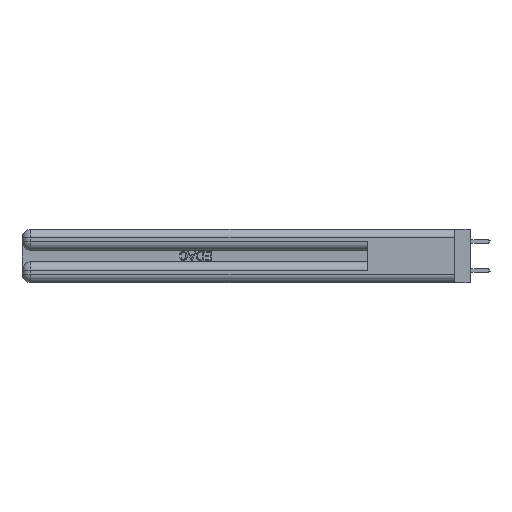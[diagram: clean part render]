
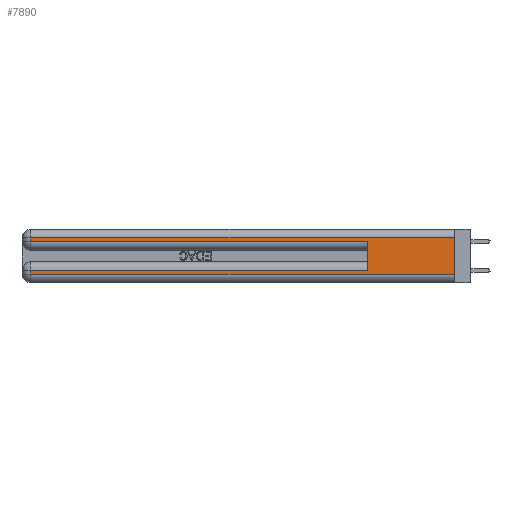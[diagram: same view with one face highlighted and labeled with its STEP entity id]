
A CAD part, left-side view. The second image highlights one B-rep face of the part: STEP entity #7890.
In plain terms, the highlighted planar face has unit normal (-1, 0, 0).
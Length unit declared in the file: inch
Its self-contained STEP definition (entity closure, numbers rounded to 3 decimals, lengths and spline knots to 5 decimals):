
#1104 = VECTOR ( 'NONE', #36062, 39.37008 ) ;
#1747 = LINE ( 'NONE', #12879, #42386 ) ;
#1796 = LINE ( 'NONE', #11357, #41329 ) ;
#2652 = DIRECTION ( 'NONE',  ( 0., 0., -1. ) ) ;
#4220 = DIRECTION ( 'NONE',  ( 0., 0., 1. ) ) ;
#4617 = VECTOR ( 'NONE', #34123, 39.37008 ) ;
#5844 = PLANE ( 'NONE',  #22096 ) ;
#7332 = LINE ( 'NONE', #20601, #35048 ) ;
#7825 = VERTEX_POINT ( 'NONE', #23229 ) ;
#7890 = ADVANCED_FACE ( 'NONE', ( #29315 ), #5844, .F. ) ;
#8463 = LINE ( 'NONE', #35904, #1104 ) ;
#9007 = DIRECTION ( 'NONE',  ( 0., 0., -1. ) ) ;
#10583 = VERTEX_POINT ( 'NONE', #43640 ) ;
#11357 = CARTESIAN_POINT ( 'NONE',  ( 0., 0., 0.085 ) ) ;
#11877 = CARTESIAN_POINT ( 'NONE',  ( 0., 2.94, 0.31 ) ) ;
#12556 = VERTEX_POINT ( 'NONE', #19531 ) ;
#12879 = CARTESIAN_POINT ( 'NONE',  ( 0., 0., 0.06 ) ) ;
#13426 = CARTESIAN_POINT ( 'NONE',  ( 0., 2.94, 0.085 ) ) ;
#14580 = ORIENTED_EDGE ( 'NONE', *, *, #31285, .T. ) ;
#15949 = ORIENTED_EDGE ( 'NONE', *, *, #45299, .F. ) ;
#16547 = LINE ( 'NONE', #38335, #45295 ) ;
#16735 = LINE ( 'NONE', #44305, #24644 ) ;
#17589 = EDGE_LOOP ( 'NONE', ( #15949, #14580, #35739, #26952, #22542, #34376, #24876, #18691 ) ) ;
#18691 = ORIENTED_EDGE ( 'NONE', *, *, #38972, .T. ) ;
#19492 = LINE ( 'NONE', #37578, #43164 ) ;
#19531 = CARTESIAN_POINT ( 'NONE',  ( 0., 0., 0.31 ) ) ;
#20601 = CARTESIAN_POINT ( 'NONE',  ( 0., 2.94, 0.37 ) ) ;
#21417 = VERTEX_POINT ( 'NONE', #11877 ) ;
#22096 = AXIS2_PLACEMENT_3D ( 'NONE', #23382, #38055, #9007 ) ;
#22542 = ORIENTED_EDGE ( 'NONE', *, *, #33859, .F. ) ;
#22879 = EDGE_CURVE ( 'NONE', #43038, #34829, #1796, .T. ) ;
#23229 = CARTESIAN_POINT ( 'NONE',  ( 0., 0., 0.06 ) ) ;
#23382 = CARTESIAN_POINT ( 'NONE',  ( 0., 0., 0.37 ) ) ;
#24644 = VECTOR ( 'NONE', #4220, 39.37008 ) ;
#24876 = ORIENTED_EDGE ( 'NONE', *, *, #25751, .T. ) ;
#25751 = EDGE_CURVE ( 'NONE', #34829, #10583, #7332, .T. ) ;
#26952 = ORIENTED_EDGE ( 'NONE', *, *, #34587, .T. ) ;
#27766 = CARTESIAN_POINT ( 'NONE',  ( 0., 0.6, 0.085 ) ) ;
#28884 = LINE ( 'NONE', #41337, #4617 ) ;
#29315 = FACE_OUTER_BOUND ( 'NONE', #17589, .T. ) ;
#30829 = VERTEX_POINT ( 'NONE', #41134 ) ;
#31285 = EDGE_CURVE ( 'NONE', #12556, #21417, #8463, .T. ) ;
#32990 = DIRECTION ( 'NONE',  ( 0., 1., 0. ) ) ;
#33859 = EDGE_CURVE ( 'NONE', #43038, #38944, #16735, .T. ) ;
#34123 = DIRECTION ( 'NONE',  ( 0., 0., -1. ) ) ;
#34376 = ORIENTED_EDGE ( 'NONE', *, *, #22879, .T. ) ;
#34587 = EDGE_CURVE ( 'NONE', #30829, #38944, #19492, .T. ) ;
#34829 = VERTEX_POINT ( 'NONE', #13426 ) ;
#34949 = DIRECTION ( 'NONE',  ( 0., -1., 0. ) ) ;
#34999 = DIRECTION ( 'NONE',  ( 0., 0., -1. ) ) ;
#35048 = VECTOR ( 'NONE', #34999, 39.37008 ) ;
#35739 = ORIENTED_EDGE ( 'NONE', *, *, #36303, .T. ) ;
#35904 = CARTESIAN_POINT ( 'NONE',  ( 0., 0., 0.31 ) ) ;
#36062 = DIRECTION ( 'NONE',  ( 0., 1., 0. ) ) ;
#36303 = EDGE_CURVE ( 'NONE', #21417, #30829, #28884, .T. ) ;
#37578 = CARTESIAN_POINT ( 'NONE',  ( 0., 0., 0.285 ) ) ;
#38055 = DIRECTION ( 'NONE',  ( 1., 0., 0. ) ) ;
#38335 = CARTESIAN_POINT ( 'NONE',  ( 0., 0., 0.37 ) ) ;
#38944 = VERTEX_POINT ( 'NONE', #41400 ) ;
#38972 = EDGE_CURVE ( 'NONE', #10583, #7825, #1747, .T. ) ;
#41024 = DIRECTION ( 'NONE',  ( 0., -1., 0. ) ) ;
#41134 = CARTESIAN_POINT ( 'NONE',  ( 0., 2.94, 0.285 ) ) ;
#41329 = VECTOR ( 'NONE', #32990, 39.37008 ) ;
#41337 = CARTESIAN_POINT ( 'NONE',  ( 0., 2.94, 0.37 ) ) ;
#41400 = CARTESIAN_POINT ( 'NONE',  ( 0., 0.6, 0.285 ) ) ;
#42386 = VECTOR ( 'NONE', #34949, 39.37008 ) ;
#43038 = VERTEX_POINT ( 'NONE', #27766 ) ;
#43164 = VECTOR ( 'NONE', #41024, 39.37008 ) ;
#43640 = CARTESIAN_POINT ( 'NONE',  ( 0., 2.94, 0.06 ) ) ;
#44305 = CARTESIAN_POINT ( 'NONE',  ( 0., 0.6, 0.145 ) ) ;
#45295 = VECTOR ( 'NONE', #2652, 39.37008 ) ;
#45299 = EDGE_CURVE ( 'NONE', #12556, #7825, #16547, .T. ) ;
